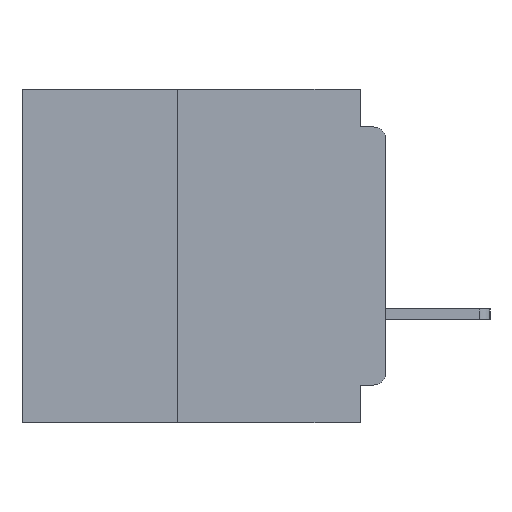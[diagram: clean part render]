
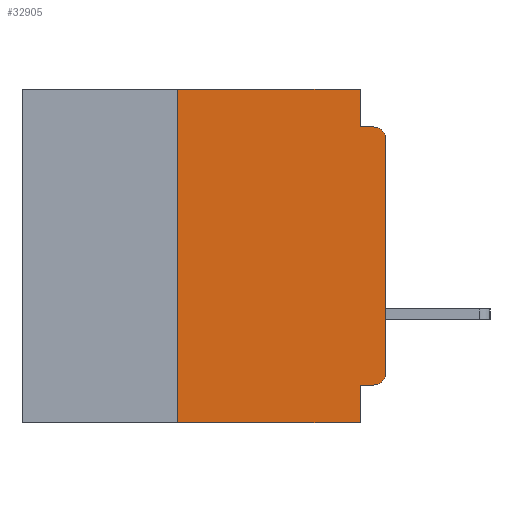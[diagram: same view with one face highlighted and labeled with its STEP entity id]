
A CAD part, left-side view. The second image highlights one B-rep face of the part: STEP entity #32905.
In plain terms, the highlighted planar face has unit normal (-1, 0, 0).
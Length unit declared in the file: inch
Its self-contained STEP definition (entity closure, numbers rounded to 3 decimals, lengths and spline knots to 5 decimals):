
#624 = CARTESIAN_POINT ( 'NONE',  ( 0., 0.015, -0.355 ) ) ;
#855 = VERTEX_POINT ( 'NONE', #3165 ) ;
#1281 = LINE ( 'NONE', #52240, #24393 ) ;
#2280 = LINE ( 'NONE', #10561, #44334 ) ;
#2509 = VECTOR ( 'NONE', #10582, 39.37008 ) ;
#2638 = EDGE_CURVE ( 'NONE', #31583, #15176, #34981, .T. ) ;
#2899 = VERTEX_POINT ( 'NONE', #624 ) ;
#3165 = CARTESIAN_POINT ( 'NONE',  ( 0., 0.031, -0.355 ) ) ;
#4461 = CARTESIAN_POINT ( 'NONE',  ( 0., 0., -0.045 ) ) ;
#5463 = VECTOR ( 'NONE', #51670, 39.37008 ) ;
#5979 = VERTEX_POINT ( 'NONE', #44974 ) ;
#6136 = VECTOR ( 'NONE', #30364, 39.37008 ) ;
#7134 = LINE ( 'NONE', #16704, #39539 ) ;
#7543 = DIRECTION ( 'NONE',  ( 0., -1., 0. ) ) ;
#7567 = VERTEX_POINT ( 'NONE', #28374 ) ;
#7954 = EDGE_CURVE ( 'NONE', #34346, #7567, #52309, .T. ) ;
#8447 = ORIENTED_EDGE ( 'NONE', *, *, #24823, .T. ) ;
#8749 = LINE ( 'NONE', #34403, #6136 ) ;
#10402 = DIRECTION ( 'NONE',  ( 0., 0., 1. ) ) ;
#10561 = CARTESIAN_POINT ( 'NONE',  ( 0., 0.031, -0.4 ) ) ;
#10582 = DIRECTION ( 'NONE',  ( 0., 0., -1. ) ) ;
#12915 = CARTESIAN_POINT ( 'NONE',  ( 0., 0.031, -0.045 ) ) ;
#13052 = VECTOR ( 'NONE', #10402, 39.37008 ) ;
#13472 = CARTESIAN_POINT ( 'NONE',  ( 0., 0., -0.06 ) ) ;
#13540 = FACE_OUTER_BOUND ( 'NONE', #35671, .T. ) ;
#13578 = CIRCLE ( 'NONE', #48216, 0.015 ) ;
#13712 = LINE ( 'NONE', #4461, #24512 ) ;
#15176 = VERTEX_POINT ( 'NONE', #12915 ) ;
#15322 = CARTESIAN_POINT ( 'NONE',  ( 0., 0.015, -0.045 ) ) ;
#15847 = DIRECTION ( 'NONE',  ( -1., 0., 0. ) ) ;
#16704 = CARTESIAN_POINT ( 'NONE',  ( 0., 0.437, 0. ) ) ;
#17148 = EDGE_CURVE ( 'NONE', #855, #23101, #2280, .T. ) ;
#21600 = AXIS2_PLACEMENT_3D ( 'NONE', #22717, #50989, #26760 ) ;
#21745 = ORIENTED_EDGE ( 'NONE', *, *, #43047, .T. ) ;
#22216 = EDGE_CURVE ( 'NONE', #2899, #855, #28467, .T. ) ;
#22717 = CARTESIAN_POINT ( 'NONE',  ( 0., 0.015, -0.06 ) ) ;
#22906 = PLANE ( 'NONE',  #29509 ) ;
#23101 = VERTEX_POINT ( 'NONE', #46297 ) ;
#23550 = ORIENTED_EDGE ( 'NONE', *, *, #49087, .T. ) ;
#24393 = VECTOR ( 'NONE', #7543, 39.37008 ) ;
#24512 = VECTOR ( 'NONE', #32919, 39.37008 ) ;
#24786 = EDGE_CURVE ( 'NONE', #2899, #5979, #13578, .T. ) ;
#24823 = EDGE_CURVE ( 'NONE', #34346, #23101, #1281, .T. ) ;
#26760 = DIRECTION ( 'NONE',  ( 0., 0., -1. ) ) ;
#26954 = DIRECTION ( 'NONE',  ( 0., 0., -1. ) ) ;
#28374 = CARTESIAN_POINT ( 'NONE',  ( 0., 0.25, 0. ) ) ;
#28467 = LINE ( 'NONE', #43545, #5463 ) ;
#29509 = AXIS2_PLACEMENT_3D ( 'NONE', #38949, #51170, #26954 ) ;
#30364 = DIRECTION ( 'NONE',  ( 0., 0., 1. ) ) ;
#31583 = VERTEX_POINT ( 'NONE', #43911 ) ;
#31606 = CIRCLE ( 'NONE', #21600, 0.015 ) ;
#32905 = ADVANCED_FACE ( 'NONE', ( #13540 ), #22906, .F. ) ;
#32919 = DIRECTION ( 'NONE',  ( 0., -1., 0. ) ) ;
#34115 = ORIENTED_EDGE ( 'NONE', *, *, #24786, .T. ) ;
#34346 = VERTEX_POINT ( 'NONE', #36294 ) ;
#34403 = CARTESIAN_POINT ( 'NONE',  ( 0., 0., 0. ) ) ;
#34804 = DIRECTION ( 'NONE',  ( 0., 0., -1. ) ) ;
#34825 = CARTESIAN_POINT ( 'NONE',  ( 0., 0.031, 0. ) ) ;
#34981 = LINE ( 'NONE', #34825, #2509 ) ;
#35671 = EDGE_LOOP ( 'NONE', ( #21745, #23550, #52624, #37936, #36401, #47456, #8447, #36503, #52775, #34115 ) ) ;
#36294 = CARTESIAN_POINT ( 'NONE',  ( 0., 0.25, -0.4 ) ) ;
#36401 = ORIENTED_EDGE ( 'NONE', *, *, #37974, .F. ) ;
#36503 = ORIENTED_EDGE ( 'NONE', *, *, #17148, .F. ) ;
#36543 = VERTEX_POINT ( 'NONE', #13472 ) ;
#37936 = ORIENTED_EDGE ( 'NONE', *, *, #2638, .F. ) ;
#37974 = EDGE_CURVE ( 'NONE', #7567, #31583, #7134, .T. ) ;
#38949 = CARTESIAN_POINT ( 'NONE',  ( 0., 0.437, 0. ) ) ;
#39539 = VECTOR ( 'NONE', #49057, 39.37008 ) ;
#40007 = CARTESIAN_POINT ( 'NONE',  ( 0., 0.015, -0.34 ) ) ;
#43047 = EDGE_CURVE ( 'NONE', #5979, #36543, #8749, .T. ) ;
#43545 = CARTESIAN_POINT ( 'NONE',  ( 0., 0., -0.355 ) ) ;
#43911 = CARTESIAN_POINT ( 'NONE',  ( 0., 0.031, 0. ) ) ;
#44116 = DIRECTION ( 'NONE',  ( 0., 0., -1. ) ) ;
#44334 = VECTOR ( 'NONE', #34804, 39.37008 ) ;
#44974 = CARTESIAN_POINT ( 'NONE',  ( 0., 0., -0.34 ) ) ;
#46297 = CARTESIAN_POINT ( 'NONE',  ( 0., 0.031, -0.4 ) ) ;
#46753 = CARTESIAN_POINT ( 'NONE',  ( 0., 0.25, -0.4 ) ) ;
#47456 = ORIENTED_EDGE ( 'NONE', *, *, #7954, .F. ) ;
#48161 = VERTEX_POINT ( 'NONE', #15322 ) ;
#48216 = AXIS2_PLACEMENT_3D ( 'NONE', #40007, #15847, #44116 ) ;
#49057 = DIRECTION ( 'NONE',  ( 0., -1., 0. ) ) ;
#49087 = EDGE_CURVE ( 'NONE', #36543, #48161, #31606, .T. ) ;
#50989 = DIRECTION ( 'NONE',  ( -1., 0., 0. ) ) ;
#51170 = DIRECTION ( 'NONE',  ( 1., 0., 0. ) ) ;
#51670 = DIRECTION ( 'NONE',  ( 0., 1., 0. ) ) ;
#52240 = CARTESIAN_POINT ( 'NONE',  ( 0., 0.437, -0.4 ) ) ;
#52309 = LINE ( 'NONE', #46753, #13052 ) ;
#52428 = EDGE_CURVE ( 'NONE', #15176, #48161, #13712, .T. ) ;
#52624 = ORIENTED_EDGE ( 'NONE', *, *, #52428, .F. ) ;
#52775 = ORIENTED_EDGE ( 'NONE', *, *, #22216, .F. ) ;
